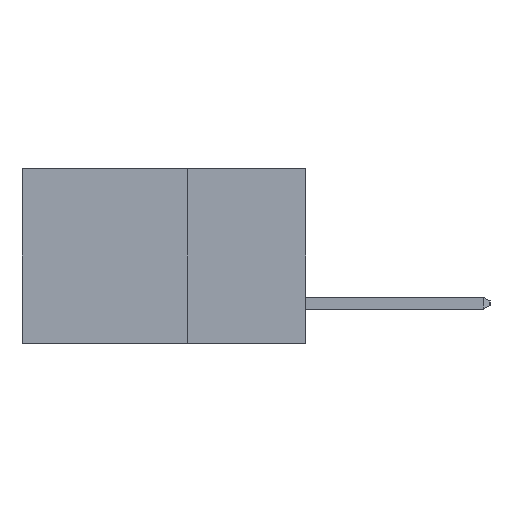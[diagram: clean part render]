
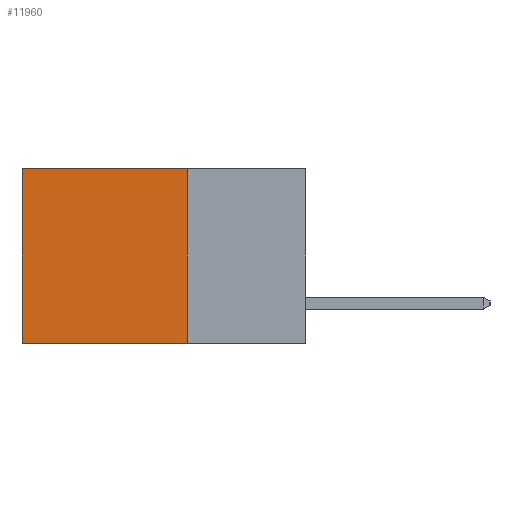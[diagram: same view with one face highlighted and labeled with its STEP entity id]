
A CAD part, left-side view. The second image highlights one B-rep face of the part: STEP entity #11960.
In plain terms, the highlighted planar face has unit normal (-1, 0, 0).
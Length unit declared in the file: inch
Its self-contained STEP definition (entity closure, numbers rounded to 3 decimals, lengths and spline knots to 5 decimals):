
#795 = CARTESIAN_POINT ( 'NONE',  ( 0.298, 0.25, 0. ) ) ;
#1139 = ORIENTED_EDGE ( 'NONE', *, *, #16913, .T. ) ;
#2304 = DIRECTION ( 'NONE',  ( 1., 0., 0. ) ) ;
#2442 = CARTESIAN_POINT ( 'NONE',  ( 0.298, 0.25, -0.37 ) ) ;
#2563 = EDGE_CURVE ( 'NONE', #16662, #2888, #3183, .T. ) ;
#2732 = VECTOR ( 'NONE', #17701, 39.37008 ) ;
#2888 = VERTEX_POINT ( 'NONE', #8207 ) ;
#3183 = LINE ( 'NONE', #16406, #2732 ) ;
#3712 = CARTESIAN_POINT ( 'NONE',  ( 0.298, 0.25, 0. ) ) ;
#4004 = DIRECTION ( 'NONE',  ( 0., 1., 0. ) ) ;
#4588 = DIRECTION ( 'NONE',  ( 0., 1., 0. ) ) ;
#4721 = ORIENTED_EDGE ( 'NONE', *, *, #16655, .F. ) ;
#6309 = VECTOR ( 'NONE', #9553, 39.37008 ) ;
#6743 = LINE ( 'NONE', #3712, #6309 ) ;
#7540 = VECTOR ( 'NONE', #4588, 39.37008 ) ;
#8183 = ORIENTED_EDGE ( 'NONE', *, *, #2563, .T. ) ;
#8207 = CARTESIAN_POINT ( 'NONE',  ( 0.298, 0.6, -0.37 ) ) ;
#8228 = VECTOR ( 'NONE', #4004, 39.37008 ) ;
#8934 = CARTESIAN_POINT ( 'NONE',  ( 0.298, 0.25, 0. ) ) ;
#9143 = CARTESIAN_POINT ( 'NONE',  ( 0.298, 0.25, -0.37 ) ) ;
#9553 = DIRECTION ( 'NONE',  ( 0., 0., -1. ) ) ;
#11483 = LINE ( 'NONE', #8934, #7540 ) ;
#11687 = VERTEX_POINT ( 'NONE', #13352 ) ;
#11901 = AXIS2_PLACEMENT_3D ( 'NONE', #795, #2304, #12597 ) ;
#11960 = ADVANCED_FACE ( 'NONE', ( #14329 ), #18318, .F. ) ;
#12405 = VERTEX_POINT ( 'NONE', #9143 ) ;
#12597 = DIRECTION ( 'NONE',  ( 0., 0., -1. ) ) ;
#12789 = CARTESIAN_POINT ( 'NONE',  ( 0.298, 0.6, 0. ) ) ;
#13352 = CARTESIAN_POINT ( 'NONE',  ( 0.298, 0.25, 0. ) ) ;
#13675 = EDGE_LOOP ( 'NONE', ( #8183, #4721, #18593, #1139 ) ) ;
#14329 = FACE_OUTER_BOUND ( 'NONE', #13675, .T. ) ;
#14480 = EDGE_CURVE ( 'NONE', #11687, #12405, #6743, .T. ) ;
#16406 = CARTESIAN_POINT ( 'NONE',  ( 0.298, 0.6, 0. ) ) ;
#16476 = LINE ( 'NONE', #2442, #8228 ) ;
#16655 = EDGE_CURVE ( 'NONE', #12405, #2888, #16476, .T. ) ;
#16662 = VERTEX_POINT ( 'NONE', #12789 ) ;
#16913 = EDGE_CURVE ( 'NONE', #11687, #16662, #11483, .T. ) ;
#17701 = DIRECTION ( 'NONE',  ( 0., 0., -1. ) ) ;
#18318 = PLANE ( 'NONE',  #11901 ) ;
#18593 = ORIENTED_EDGE ( 'NONE', *, *, #14480, .F. ) ;
